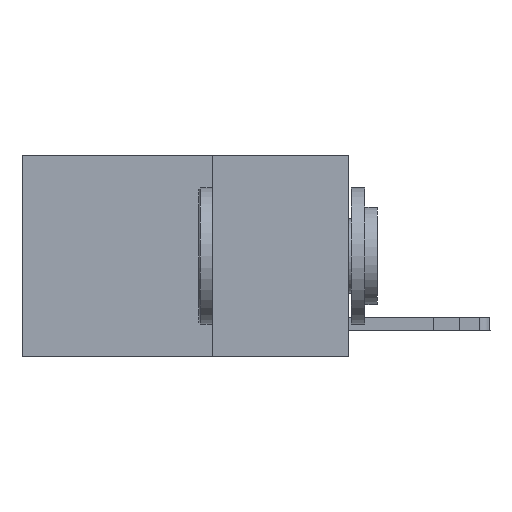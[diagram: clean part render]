
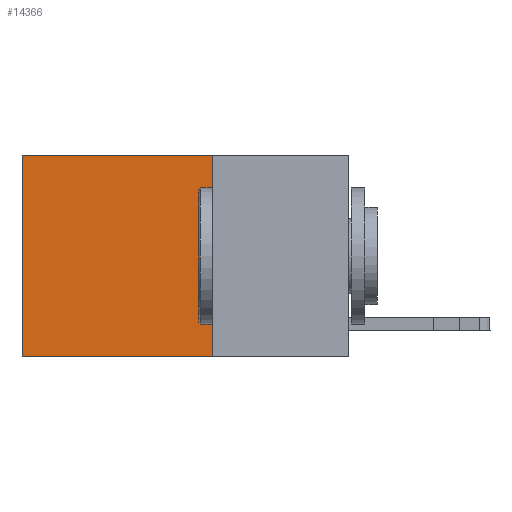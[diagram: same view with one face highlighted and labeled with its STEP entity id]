
A CAD part, left-side view. The second image highlights one B-rep face of the part: STEP entity #14366.
In plain terms, the highlighted planar face has unit normal (-1, 0, 0).
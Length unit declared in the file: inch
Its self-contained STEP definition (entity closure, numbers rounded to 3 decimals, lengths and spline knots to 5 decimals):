
#790 = VECTOR ( 'NONE', #13506, 39.37008 ) ;
#1155 = DIRECTION ( 'NONE',  ( 0., 0., -1. ) ) ;
#1420 = CARTESIAN_POINT ( 'NONE',  ( 0.2625, 0.25, 0. ) ) ;
#1668 = VECTOR ( 'NONE', #4486, 39.37008 ) ;
#2274 = LINE ( 'NONE', #8042, #1668 ) ;
#2329 = LINE ( 'NONE', #23913, #24644 ) ;
#2458 = DIRECTION ( 'NONE',  ( 0., 0., -1. ) ) ;
#3230 = LINE ( 'NONE', #17117, #15927 ) ;
#3789 = CARTESIAN_POINT ( 'NONE',  ( 0.2625, 0.25, -0.37 ) ) ;
#4486 = DIRECTION ( 'NONE',  ( 0., 1., 0. ) ) ;
#4954 = EDGE_CURVE ( 'NONE', #20140, #22468, #11427, .T. ) ;
#6626 = EDGE_LOOP ( 'NONE', ( #23790, #17670, #20500, #12866 ) ) ;
#8042 = CARTESIAN_POINT ( 'NONE',  ( 0.2625, 0.25, -0.37 ) ) ;
#8078 = EDGE_CURVE ( 'NONE', #20140, #11259, #3230, .T. ) ;
#9234 = DIRECTION ( 'NONE',  ( 1., 0., 0. ) ) ;
#11168 = DIRECTION ( 'NONE',  ( 0., 1., 0. ) ) ;
#11259 = VERTEX_POINT ( 'NONE', #22434 ) ;
#11427 = LINE ( 'NONE', #1420, #790 ) ;
#12866 = ORIENTED_EDGE ( 'NONE', *, *, #8078, .T. ) ;
#13331 = AXIS2_PLACEMENT_3D ( 'NONE', #21389, #9234, #1155 ) ;
#13506 = DIRECTION ( 'NONE',  ( 0., 0., -1. ) ) ;
#14366 = ADVANCED_FACE ( 'NONE', ( #18934 ), #17355, .F. ) ;
#15646 = EDGE_CURVE ( 'NONE', #11259, #18772, #2329, .T. ) ;
#15927 = VECTOR ( 'NONE', #11168, 39.37008 ) ;
#15992 = CARTESIAN_POINT ( 'NONE',  ( 0.2625, 0.6, -0.37 ) ) ;
#17117 = CARTESIAN_POINT ( 'NONE',  ( 0.2625, 0.25, 0. ) ) ;
#17355 = PLANE ( 'NONE',  #13331 ) ;
#17670 = ORIENTED_EDGE ( 'NONE', *, *, #19126, .F. ) ;
#18772 = VERTEX_POINT ( 'NONE', #15992 ) ;
#18792 = CARTESIAN_POINT ( 'NONE',  ( 0.2625, 0.25, 0. ) ) ;
#18934 = FACE_OUTER_BOUND ( 'NONE', #6626, .T. ) ;
#19126 = EDGE_CURVE ( 'NONE', #22468, #18772, #2274, .T. ) ;
#20140 = VERTEX_POINT ( 'NONE', #18792 ) ;
#20500 = ORIENTED_EDGE ( 'NONE', *, *, #4954, .F. ) ;
#21389 = CARTESIAN_POINT ( 'NONE',  ( 0.2625, 0.25, 0. ) ) ;
#22434 = CARTESIAN_POINT ( 'NONE',  ( 0.2625, 0.6, 0. ) ) ;
#22468 = VERTEX_POINT ( 'NONE', #3789 ) ;
#23790 = ORIENTED_EDGE ( 'NONE', *, *, #15646, .T. ) ;
#23913 = CARTESIAN_POINT ( 'NONE',  ( 0.2625, 0.6, 0. ) ) ;
#24644 = VECTOR ( 'NONE', #2458, 39.37008 ) ;
